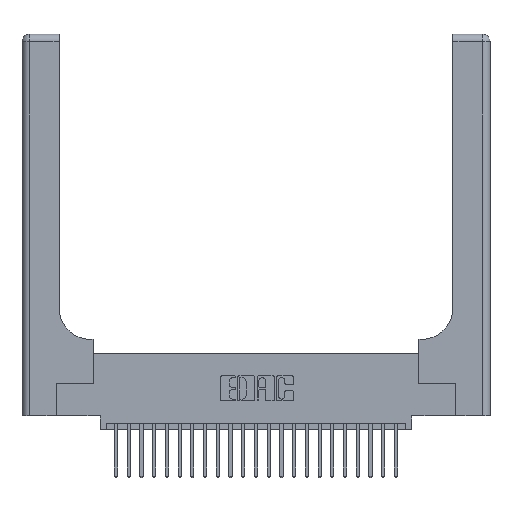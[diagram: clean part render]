
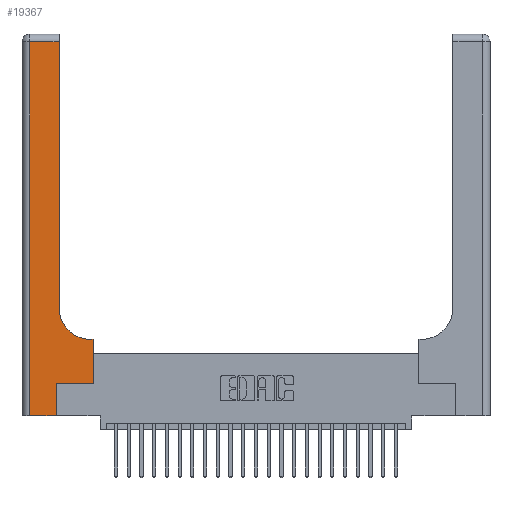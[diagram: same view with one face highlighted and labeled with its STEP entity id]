
A CAD part, top view. The second image highlights one B-rep face of the part: STEP entity #19367.
In plain terms, the highlighted planar face has unit normal (0, 0, 1).
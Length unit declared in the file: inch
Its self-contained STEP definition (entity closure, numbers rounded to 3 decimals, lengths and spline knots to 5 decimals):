
#283 = EDGE_CURVE ( 'NONE', #19891, #18739, #19507, .T. ) ;
#361 = CARTESIAN_POINT ( 'NONE',  ( 0.269, 0.25, 0.37 ) ) ;
#564 = VERTEX_POINT ( 'NONE', #21772 ) ;
#622 = DIRECTION ( 'NONE',  ( 1., 0., 0. ) ) ;
#632 = DIRECTION ( 'NONE',  ( -1., 0., 0. ) ) ;
#1279 = DIRECTION ( 'NONE',  ( -1., 0., 0. ) ) ;
#1304 = ORIENTED_EDGE ( 'NONE', *, *, #18376, .T. ) ;
#1397 = EDGE_LOOP ( 'NONE', ( #13552, #17664, #19851, #7764, #1304, #13747, #11756, #21300, #24773 ) ) ;
#1405 = CARTESIAN_POINT ( 'NONE',  ( 0.5585, 0.6, 0.37 ) ) ;
#1516 = AXIS2_PLACEMENT_3D ( 'NONE', #12955, #10610, #632 ) ;
#1542 = LINE ( 'NONE', #20882, #9968 ) ;
#1919 = CARTESIAN_POINT ( 'NONE',  ( 0.2915, 2.94, 0.37 ) ) ;
#2501 = CARTESIAN_POINT ( 'NONE',  ( 0.5415, 0.6, 0.37 ) ) ;
#2978 = CARTESIAN_POINT ( 'NONE',  ( 0.2915, 3., 0.37 ) ) ;
#3047 = DIRECTION ( 'NONE',  ( 1., 0., 0. ) ) ;
#3060 = VERTEX_POINT ( 'NONE', #17688 ) ;
#3290 = EDGE_CURVE ( 'NONE', #6149, #19891, #13999, .T. ) ;
#3441 = LINE ( 'NONE', #13320, #6541 ) ;
#3759 = DIRECTION ( 'NONE',  ( -1., 0., 0. ) ) ;
#4104 = VECTOR ( 'NONE', #14935, 39.37008 ) ;
#5481 = CARTESIAN_POINT ( 'NONE',  ( 0.269, 0., 0.37 ) ) ;
#6018 = VECTOR ( 'NONE', #3047, 39.37008 ) ;
#6149 = VERTEX_POINT ( 'NONE', #22518 ) ;
#6488 = VECTOR ( 'NONE', #3759, 39.37008 ) ;
#6541 = VECTOR ( 'NONE', #1279, 39.37008 ) ;
#6912 = CARTESIAN_POINT ( 'NONE',  ( 0.06, 0., 0.37 ) ) ;
#7764 = ORIENTED_EDGE ( 'NONE', *, *, #283, .T. ) ;
#8147 = LINE ( 'NONE', #2978, #4104 ) ;
#8305 = DIRECTION ( 'NONE',  ( 0., -1., 0. ) ) ;
#9600 = EDGE_CURVE ( 'NONE', #13368, #21767, #8147, .T. ) ;
#9889 = CARTESIAN_POINT ( 'NONE',  ( 0.2915, 0.85, 0.37 ) ) ;
#9968 = VECTOR ( 'NONE', #25008, 39.37008 ) ;
#10221 = CARTESIAN_POINT ( 'NONE',  ( 0.06, 3., 0.37 ) ) ;
#10610 = DIRECTION ( 'NONE',  ( 0., 0., -1. ) ) ;
#11756 = ORIENTED_EDGE ( 'NONE', *, *, #16688, .T. ) ;
#12757 = VECTOR ( 'NONE', #16413, 39.37008 ) ;
#12955 = CARTESIAN_POINT ( 'NONE',  ( 0., 3., 0.37 ) ) ;
#13320 = CARTESIAN_POINT ( 'NONE',  ( 0., 2.94, 0.37 ) ) ;
#13368 = VERTEX_POINT ( 'NONE', #9889 ) ;
#13552 = ORIENTED_EDGE ( 'NONE', *, *, #9600, .T. ) ;
#13747 = ORIENTED_EDGE ( 'NONE', *, *, #16544, .T. ) ;
#13999 = LINE ( 'NONE', #10221, #22154 ) ;
#14895 = CARTESIAN_POINT ( 'NONE',  ( 0.269, 0., 0.37 ) ) ;
#14935 = DIRECTION ( 'NONE',  ( 0., 1., 0. ) ) ;
#15654 = VERTEX_POINT ( 'NONE', #1405 ) ;
#16125 = AXIS2_PLACEMENT_3D ( 'NONE', #18512, #18684, #622 ) ;
#16413 = DIRECTION ( 'NONE',  ( 1., 0., 0. ) ) ;
#16544 = EDGE_CURVE ( 'NONE', #564, #3060, #21583, .T. ) ;
#16688 = EDGE_CURVE ( 'NONE', #3060, #15654, #1542, .T. ) ;
#16721 = EDGE_CURVE ( 'NONE', #21767, #6149, #3441, .T. ) ;
#16843 = VECTOR ( 'NONE', #18947, 39.37008 ) ;
#17159 = LINE ( 'NONE', #14895, #16843 ) ;
#17405 = EDGE_CURVE ( 'NONE', #15654, #25352, #24377, .T. ) ;
#17620 = FACE_OUTER_BOUND ( 'NONE', #1397, .T. ) ;
#17664 = ORIENTED_EDGE ( 'NONE', *, *, #16721, .T. ) ;
#17688 = CARTESIAN_POINT ( 'NONE',  ( 0.5585, 0.25, 0.37 ) ) ;
#18037 = CARTESIAN_POINT ( 'NONE',  ( 0.2915, 0.6, 0.37 ) ) ;
#18376 = EDGE_CURVE ( 'NONE', #18739, #564, #17159, .T. ) ;
#18512 = CARTESIAN_POINT ( 'NONE',  ( 0.5415, 0.85, 0.37 ) ) ;
#18609 = PLANE ( 'NONE',  #1516 ) ;
#18684 = DIRECTION ( 'NONE',  ( 0., 0., -1. ) ) ;
#18739 = VERTEX_POINT ( 'NONE', #5481 ) ;
#18947 = DIRECTION ( 'NONE',  ( 0., 1., 0. ) ) ;
#19367 = ADVANCED_FACE ( 'NONE', ( #17620 ), #18609, .F. ) ;
#19473 = CIRCLE ( 'NONE', #16125, 0.25 ) ;
#19507 = LINE ( 'NONE', #25098, #6018 ) ;
#19851 = ORIENTED_EDGE ( 'NONE', *, *, #3290, .T. ) ;
#19891 = VERTEX_POINT ( 'NONE', #6912 ) ;
#20277 = EDGE_CURVE ( 'NONE', #25352, #13368, #19473, .T. ) ;
#20882 = CARTESIAN_POINT ( 'NONE',  ( 0.5585, 0.25, 0.37 ) ) ;
#21300 = ORIENTED_EDGE ( 'NONE', *, *, #17405, .T. ) ;
#21583 = LINE ( 'NONE', #361, #12757 ) ;
#21767 = VERTEX_POINT ( 'NONE', #1919 ) ;
#21772 = CARTESIAN_POINT ( 'NONE',  ( 0.269, 0.25, 0.37 ) ) ;
#22154 = VECTOR ( 'NONE', #8305, 39.37008 ) ;
#22518 = CARTESIAN_POINT ( 'NONE',  ( 0.06, 2.94, 0.37 ) ) ;
#24377 = LINE ( 'NONE', #18037, #6488 ) ;
#24773 = ORIENTED_EDGE ( 'NONE', *, *, #20277, .T. ) ;
#25008 = DIRECTION ( 'NONE',  ( 0., 1., 0. ) ) ;
#25098 = CARTESIAN_POINT ( 'NONE',  ( 0., 0., 0.37 ) ) ;
#25352 = VERTEX_POINT ( 'NONE', #2501 ) ;
